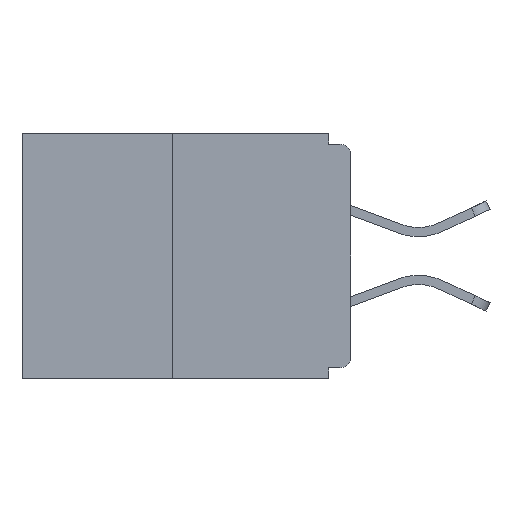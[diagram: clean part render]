
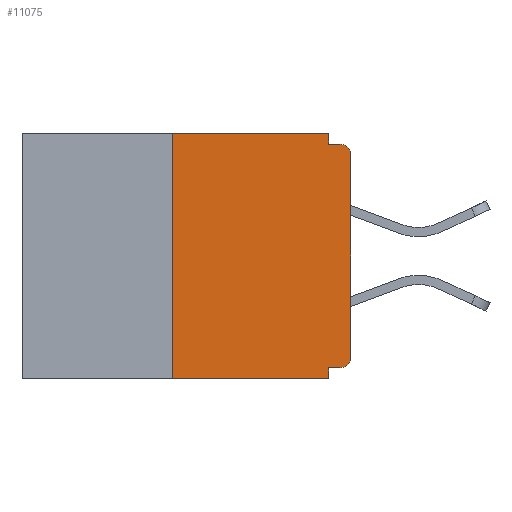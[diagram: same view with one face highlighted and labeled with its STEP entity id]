
A CAD part, left-side view. The second image highlights one B-rep face of the part: STEP entity #11075.
In plain terms, the highlighted planar face has unit normal (-1, 0, 0).
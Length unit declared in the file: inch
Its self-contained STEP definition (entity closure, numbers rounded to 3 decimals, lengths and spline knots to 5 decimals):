
#332 = CARTESIAN_POINT ( 'NONE',  ( 0., 0.46, 0. ) ) ;
#490 = ORIENTED_EDGE ( 'NONE', *, *, #14696, .T. ) ;
#995 = CARTESIAN_POINT ( 'NONE',  ( 0., 0.031, 0. ) ) ;
#1058 = AXIS2_PLACEMENT_3D ( 'NONE', #1812, #3666, #5621 ) ;
#1070 = CARTESIAN_POINT ( 'NONE',  ( 0., 0., -0.313 ) ) ;
#1285 = VERTEX_POINT ( 'NONE', #18825 ) ;
#1467 = VERTEX_POINT ( 'NONE', #23883 ) ;
#1812 = CARTESIAN_POINT ( 'NONE',  ( 0., 0.015, -0.03 ) ) ;
#2364 = LINE ( 'NONE', #11983, #9936 ) ;
#2608 = VERTEX_POINT ( 'NONE', #1070 ) ;
#3118 = LINE ( 'NONE', #3592, #4054 ) ;
#3561 = DIRECTION ( 'NONE',  ( 0., 1., 0. ) ) ;
#3592 = CARTESIAN_POINT ( 'NONE',  ( 0., 0., -0.015 ) ) ;
#3650 = CARTESIAN_POINT ( 'NONE',  ( 0., 0.015, -0.015 ) ) ;
#3666 = DIRECTION ( 'NONE',  ( -1., 0., 0. ) ) ;
#3814 = CARTESIAN_POINT ( 'NONE',  ( 0., 0.031, -0.015 ) ) ;
#3844 = CIRCLE ( 'NONE', #5329, 0.015 ) ;
#3955 = VECTOR ( 'NONE', #3561, 39.37008 ) ;
#4054 = VECTOR ( 'NONE', #11447, 39.37008 ) ;
#4268 = ORIENTED_EDGE ( 'NONE', *, *, #9237, .F. ) ;
#4657 = LINE ( 'NONE', #19510, #11330 ) ;
#5329 = AXIS2_PLACEMENT_3D ( 'NONE', #16034, #18267, #20107 ) ;
#5574 = VECTOR ( 'NONE', #24928, 39.37008 ) ;
#5585 = EDGE_CURVE ( 'NONE', #17341, #8065, #22938, .T. ) ;
#5621 = DIRECTION ( 'NONE',  ( 0., 0., -1. ) ) ;
#5673 = ORIENTED_EDGE ( 'NONE', *, *, #23914, .T. ) ;
#5918 = LINE ( 'NONE', #20551, #13750 ) ;
#5997 = DIRECTION ( 'NONE',  ( 0., -1., 0. ) ) ;
#6033 = AXIS2_PLACEMENT_3D ( 'NONE', #332, #10208, #13841 ) ;
#6442 = LINE ( 'NONE', #7590, #5574 ) ;
#7381 = CARTESIAN_POINT ( 'NONE',  ( 0., 0., -0.328 ) ) ;
#7590 = CARTESIAN_POINT ( 'NONE',  ( 0., 0.031, 0. ) ) ;
#7920 = VERTEX_POINT ( 'NONE', #3814 ) ;
#8065 = VERTEX_POINT ( 'NONE', #23444 ) ;
#8125 = EDGE_CURVE ( 'NONE', #17341, #2608, #3844, .T. ) ;
#8142 = CIRCLE ( 'NONE', #1058, 0.015 ) ;
#9237 = EDGE_CURVE ( 'NONE', #8065, #20534, #5918, .T. ) ;
#9679 = VECTOR ( 'NONE', #12649, 39.37008 ) ;
#9927 = EDGE_CURVE ( 'NONE', #7920, #22872, #3118, .T. ) ;
#9936 = VECTOR ( 'NONE', #23628, 39.37008 ) ;
#10018 = CARTESIAN_POINT ( 'NONE',  ( 0., 0.015, -0.328 ) ) ;
#10208 = DIRECTION ( 'NONE',  ( 1., 0., 0. ) ) ;
#10297 = EDGE_CURVE ( 'NONE', #18672, #7920, #6442, .T. ) ;
#11075 = ADVANCED_FACE ( 'NONE', ( #11961 ), #23435, .F. ) ;
#11330 = VECTOR ( 'NONE', #5997, 39.37008 ) ;
#11447 = DIRECTION ( 'NONE',  ( 0., -1., 0. ) ) ;
#11791 = EDGE_LOOP ( 'NONE', ( #16381, #22428, #5673, #4268, #14194, #16720, #19419, #490, #19966, #11988 ) ) ;
#11961 = FACE_OUTER_BOUND ( 'NONE', #11791, .T. ) ;
#11983 = CARTESIAN_POINT ( 'NONE',  ( 0., 0.25, 0. ) ) ;
#11988 = ORIENTED_EDGE ( 'NONE', *, *, #10297, .F. ) ;
#12615 = LINE ( 'NONE', #22426, #15069 ) ;
#12649 = DIRECTION ( 'NONE',  ( 0., -1., 0. ) ) ;
#13750 = VECTOR ( 'NONE', #20469, 39.37008 ) ;
#13841 = DIRECTION ( 'NONE',  ( 0., 0., -1. ) ) ;
#14194 = ORIENTED_EDGE ( 'NONE', *, *, #5585, .F. ) ;
#14696 = EDGE_CURVE ( 'NONE', #1467, #22872, #8142, .T. ) ;
#14890 = EDGE_CURVE ( 'NONE', #2608, #1467, #12615, .T. ) ;
#15069 = VECTOR ( 'NONE', #20307, 39.37008 ) ;
#15657 = EDGE_CURVE ( 'NONE', #1285, #23235, #2364, .T. ) ;
#16034 = CARTESIAN_POINT ( 'NONE',  ( 0., 0.015, -0.313 ) ) ;
#16381 = ORIENTED_EDGE ( 'NONE', *, *, #21008, .F. ) ;
#16453 = CARTESIAN_POINT ( 'NONE',  ( 0., 0.46, 0. ) ) ;
#16720 = ORIENTED_EDGE ( 'NONE', *, *, #8125, .T. ) ;
#16898 = CARTESIAN_POINT ( 'NONE',  ( 0., 0.031, -0.343 ) ) ;
#17341 = VERTEX_POINT ( 'NONE', #10018 ) ;
#18267 = DIRECTION ( 'NONE',  ( -1., 0., 0. ) ) ;
#18672 = VERTEX_POINT ( 'NONE', #995 ) ;
#18825 = CARTESIAN_POINT ( 'NONE',  ( 0., 0.25, -0.343 ) ) ;
#19419 = ORIENTED_EDGE ( 'NONE', *, *, #14890, .T. ) ;
#19510 = CARTESIAN_POINT ( 'NONE',  ( 0., 0.46, -0.343 ) ) ;
#19966 = ORIENTED_EDGE ( 'NONE', *, *, #9927, .F. ) ;
#20107 = DIRECTION ( 'NONE',  ( 0., 0., -1. ) ) ;
#20307 = DIRECTION ( 'NONE',  ( 0., 0., 1. ) ) ;
#20469 = DIRECTION ( 'NONE',  ( 0., 0., -1. ) ) ;
#20534 = VERTEX_POINT ( 'NONE', #16898 ) ;
#20551 = CARTESIAN_POINT ( 'NONE',  ( 0., 0.031, -0.343 ) ) ;
#21008 = EDGE_CURVE ( 'NONE', #23235, #18672, #21393, .T. ) ;
#21393 = LINE ( 'NONE', #16453, #9679 ) ;
#21461 = CARTESIAN_POINT ( 'NONE',  ( 0., 0.25, 0. ) ) ;
#22426 = CARTESIAN_POINT ( 'NONE',  ( 0., 0., 0. ) ) ;
#22428 = ORIENTED_EDGE ( 'NONE', *, *, #15657, .F. ) ;
#22872 = VERTEX_POINT ( 'NONE', #3650 ) ;
#22938 = LINE ( 'NONE', #7381, #3955 ) ;
#23235 = VERTEX_POINT ( 'NONE', #21461 ) ;
#23435 = PLANE ( 'NONE',  #6033 ) ;
#23444 = CARTESIAN_POINT ( 'NONE',  ( 0., 0.031, -0.328 ) ) ;
#23628 = DIRECTION ( 'NONE',  ( 0., 0., 1. ) ) ;
#23883 = CARTESIAN_POINT ( 'NONE',  ( 0., 0., -0.03 ) ) ;
#23914 = EDGE_CURVE ( 'NONE', #1285, #20534, #4657, .T. ) ;
#24928 = DIRECTION ( 'NONE',  ( 0., 0., -1. ) ) ;
